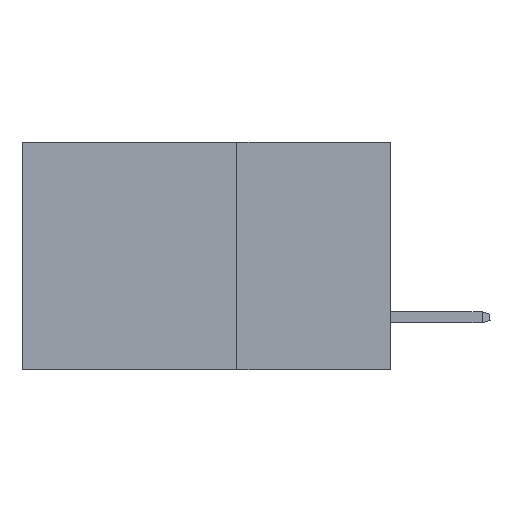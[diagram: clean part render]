
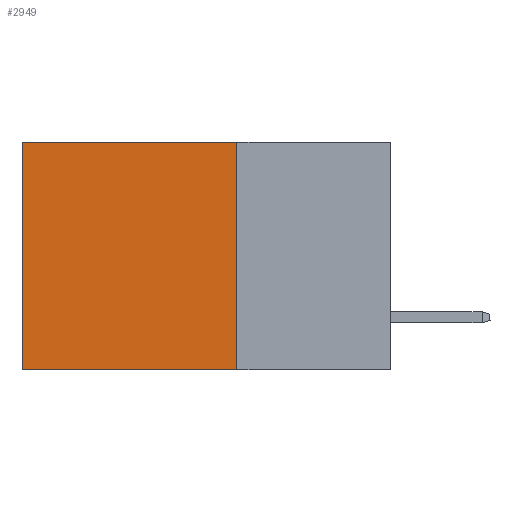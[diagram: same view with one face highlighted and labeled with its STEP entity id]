
A CAD part, left-side view. The second image highlights one B-rep face of the part: STEP entity #2949.
In plain terms, the highlighted planar face has unit normal (-1, 0, 0).
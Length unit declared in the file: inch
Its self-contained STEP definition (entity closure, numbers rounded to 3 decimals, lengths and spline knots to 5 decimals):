
#1726 = ORIENTED_EDGE ( 'NONE', *, *, #26055, .F. ) ;
#2949 = ADVANCED_FACE ( 'NONE', ( #3976 ), #7502, .F. ) ;
#3976 = FACE_OUTER_BOUND ( 'NONE', #19050, .T. ) ;
#6278 = CARTESIAN_POINT ( 'NONE',  ( 0.2875, 0.25, 0. ) ) ;
#6642 = EDGE_CURVE ( 'NONE', #30440, #9488, #23236, .T. ) ;
#6763 = ORIENTED_EDGE ( 'NONE', *, *, #7713, .T. ) ;
#6881 = DIRECTION ( 'NONE',  ( 0., 1., 0. ) ) ;
#7098 = VECTOR ( 'NONE', #12695, 39.37008 ) ;
#7502 = PLANE ( 'NONE',  #22324 ) ;
#7713 = EDGE_CURVE ( 'NONE', #14575, #24823, #31533, .T. ) ;
#8476 = CARTESIAN_POINT ( 'NONE',  ( 0.2875, 0.25, 0. ) ) ;
#8533 = LINE ( 'NONE', #31517, #26873 ) ;
#9488 = VERTEX_POINT ( 'NONE', #22520 ) ;
#9855 = CARTESIAN_POINT ( 'NONE',  ( 0.2875, 0.25, 0. ) ) ;
#10200 = VECTOR ( 'NONE', #22951, 39.37008 ) ;
#11422 = CARTESIAN_POINT ( 'NONE',  ( 0.2875, 0.6, -0.37 ) ) ;
#11968 = EDGE_CURVE ( 'NONE', #30440, #14575, #16741, .T. ) ;
#12695 = DIRECTION ( 'NONE',  ( 0., 0., -1. ) ) ;
#14575 = VERTEX_POINT ( 'NONE', #26280 ) ;
#14754 = DIRECTION ( 'NONE',  ( 1., 0., 0. ) ) ;
#16741 = LINE ( 'NONE', #9855, #22465 ) ;
#19050 = EDGE_LOOP ( 'NONE', ( #6763, #1726, #22691, #24553 ) ) ;
#22324 = AXIS2_PLACEMENT_3D ( 'NONE', #29196, #14754, #31637 ) ;
#22465 = VECTOR ( 'NONE', #27272, 39.37008 ) ;
#22520 = CARTESIAN_POINT ( 'NONE',  ( 0.2875, 0.25, -0.37 ) ) ;
#22691 = ORIENTED_EDGE ( 'NONE', *, *, #6642, .F. ) ;
#22951 = DIRECTION ( 'NONE',  ( 0., 0., -1. ) ) ;
#23236 = LINE ( 'NONE', #6278, #10200 ) ;
#24553 = ORIENTED_EDGE ( 'NONE', *, *, #11968, .T. ) ;
#24823 = VERTEX_POINT ( 'NONE', #11422 ) ;
#26055 = EDGE_CURVE ( 'NONE', #9488, #24823, #8533, .T. ) ;
#26280 = CARTESIAN_POINT ( 'NONE',  ( 0.2875, 0.6, 0. ) ) ;
#26873 = VECTOR ( 'NONE', #6881, 39.37008 ) ;
#27272 = DIRECTION ( 'NONE',  ( 0., 1., 0. ) ) ;
#27366 = CARTESIAN_POINT ( 'NONE',  ( 0.2875, 0.6, 0. ) ) ;
#29196 = CARTESIAN_POINT ( 'NONE',  ( 0.2875, 0.25, 0. ) ) ;
#30440 = VERTEX_POINT ( 'NONE', #8476 ) ;
#31517 = CARTESIAN_POINT ( 'NONE',  ( 0.2875, 0.25, -0.37 ) ) ;
#31533 = LINE ( 'NONE', #27366, #7098 ) ;
#31637 = DIRECTION ( 'NONE',  ( 0., 0., -1. ) ) ;
